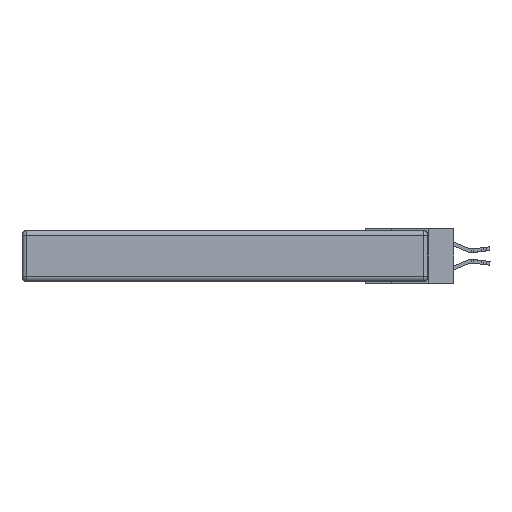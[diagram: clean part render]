
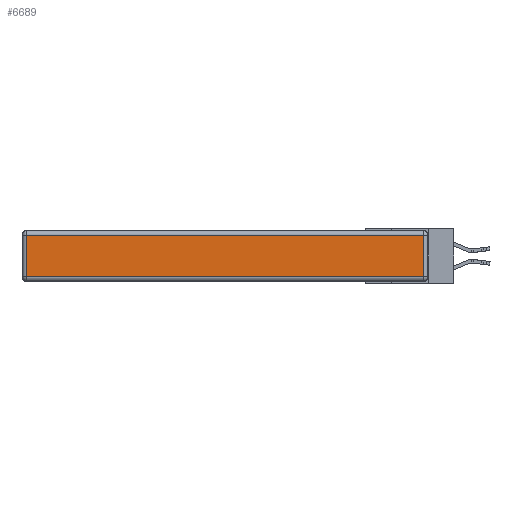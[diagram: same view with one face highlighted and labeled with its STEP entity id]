
A CAD part, left-side view. The second image highlights one B-rep face of the part: STEP entity #6689.
In plain terms, the highlighted planar face has unit normal (-1, 0, 0).
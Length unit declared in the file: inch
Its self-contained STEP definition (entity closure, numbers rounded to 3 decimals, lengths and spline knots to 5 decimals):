
#31 = LINE ( 'NONE', #17442, #28698 ) ;
#1274 = EDGE_LOOP ( 'NONE', ( #27066, #11719, #21757, #9087 ) ) ;
#1405 = CARTESIAN_POINT ( 'NONE',  ( 0., 0.03, -0.03 ) ) ;
#1978 = DIRECTION ( 'NONE',  ( 0., 1., 0. ) ) ;
#3916 = LINE ( 'NONE', #26986, #10069 ) ;
#5173 = DIRECTION ( 'NONE',  ( 0., 0., 1. ) ) ;
#5651 = VERTEX_POINT ( 'NONE', #17116 ) ;
#6225 = EDGE_CURVE ( 'NONE', #29844, #27137, #3916, .T. ) ;
#6332 = FACE_OUTER_BOUND ( 'NONE', #1274, .T. ) ;
#6662 = CARTESIAN_POINT ( 'NONE',  ( 0., 0.03, -0.313 ) ) ;
#6689 = ADVANCED_FACE ( 'NONE', ( #6332 ), #25315, .T. ) ;
#8736 = DIRECTION ( 'NONE',  ( 0., 0., 1. ) ) ;
#9087 = ORIENTED_EDGE ( 'NONE', *, *, #10562, .T. ) ;
#10069 = VECTOR ( 'NONE', #8736, 39.37008 ) ;
#10562 = EDGE_CURVE ( 'NONE', #5651, #13567, #29677, .T. ) ;
#10573 = DIRECTION ( 'NONE',  ( -1., 0., 0. ) ) ;
#11719 = ORIENTED_EDGE ( 'NONE', *, *, #6225, .T. ) ;
#12218 = AXIS2_PLACEMENT_3D ( 'NONE', #33043, #10573, #5173 ) ;
#12220 = DIRECTION ( 'NONE',  ( 0., 0., -1. ) ) ;
#13101 = EDGE_CURVE ( 'NONE', #27137, #5651, #31, .T. ) ;
#13567 = VERTEX_POINT ( 'NONE', #28639 ) ;
#17116 = CARTESIAN_POINT ( 'NONE',  ( 0., 2.72, -0.03 ) ) ;
#17442 = CARTESIAN_POINT ( 'NONE',  ( 0., 2.75, -0.03 ) ) ;
#17810 = VECTOR ( 'NONE', #17878, 39.37008 ) ;
#17878 = DIRECTION ( 'NONE',  ( 0., -1., 0. ) ) ;
#19520 = VECTOR ( 'NONE', #12220, 39.37008 ) ;
#20610 = CARTESIAN_POINT ( 'NONE',  ( 0., 0., -0.313 ) ) ;
#21757 = ORIENTED_EDGE ( 'NONE', *, *, #13101, .T. ) ;
#24563 = EDGE_CURVE ( 'NONE', #13567, #29844, #33720, .T. ) ;
#25315 = PLANE ( 'NONE',  #12218 ) ;
#26986 = CARTESIAN_POINT ( 'NONE',  ( 0., 0.03, -0.343 ) ) ;
#27066 = ORIENTED_EDGE ( 'NONE', *, *, #24563, .T. ) ;
#27137 = VERTEX_POINT ( 'NONE', #1405 ) ;
#28639 = CARTESIAN_POINT ( 'NONE',  ( 0., 2.72, -0.313 ) ) ;
#28698 = VECTOR ( 'NONE', #1978, 39.37008 ) ;
#29677 = LINE ( 'NONE', #32982, #19520 ) ;
#29844 = VERTEX_POINT ( 'NONE', #6662 ) ;
#32982 = CARTESIAN_POINT ( 'NONE',  ( 0., 2.72, -0.343 ) ) ;
#33043 = CARTESIAN_POINT ( 'NONE',  ( 0., 0., -0.343 ) ) ;
#33720 = LINE ( 'NONE', #20610, #17810 ) ;
